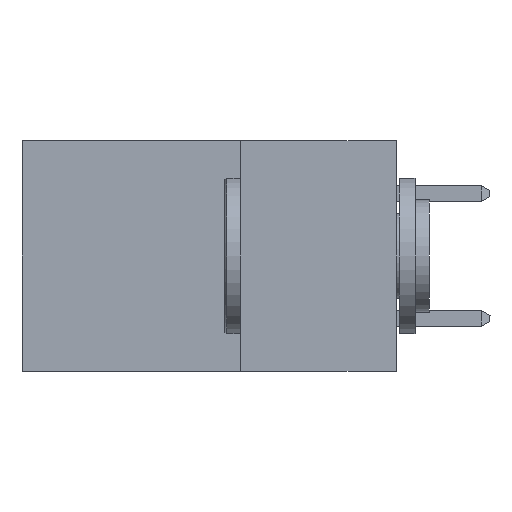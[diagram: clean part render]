
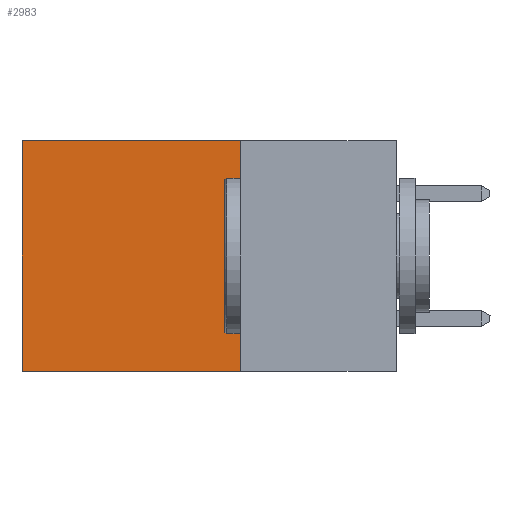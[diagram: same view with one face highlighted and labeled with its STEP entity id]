
A CAD part, left-side view. The second image highlights one B-rep face of the part: STEP entity #2983.
In plain terms, the highlighted planar face has unit normal (-1, 0, 0).
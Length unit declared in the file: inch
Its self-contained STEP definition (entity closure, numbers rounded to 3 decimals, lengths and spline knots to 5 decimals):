
#425 = EDGE_CURVE ( 'NONE', #15048, #3591, #4160, .T. ) ;
#958 = PLANE ( 'NONE',  #8337 ) ;
#1347 = EDGE_CURVE ( 'NONE', #12114, #5722, #8080, .T. ) ;
#1470 = FACE_OUTER_BOUND ( 'NONE', #16190, .T. ) ;
#1978 = CARTESIAN_POINT ( 'NONE',  ( 0.298, 0.25, 0. ) ) ;
#2418 = CARTESIAN_POINT ( 'NONE',  ( 0.298, 0.25, -0.37 ) ) ;
#2603 = VECTOR ( 'NONE', #12173, 39.37008 ) ;
#2983 = ADVANCED_FACE ( 'NONE', ( #1470 ), #958, .F. ) ;
#3263 = CARTESIAN_POINT ( 'NONE',  ( 0.298, 0.25, 0. ) ) ;
#3385 = ORIENTED_EDGE ( 'NONE', *, *, #1347, .T. ) ;
#3591 = VERTEX_POINT ( 'NONE', #10988 ) ;
#3850 = EDGE_CURVE ( 'NONE', #5722, #3591, #8456, .T. ) ;
#4106 = ORIENTED_EDGE ( 'NONE', *, *, #3850, .T. ) ;
#4160 = LINE ( 'NONE', #8777, #6154 ) ;
#4878 = ORIENTED_EDGE ( 'NONE', *, *, #15898, .F. ) ;
#5058 = DIRECTION ( 'NONE',  ( 0., 0., -1. ) ) ;
#5125 = CARTESIAN_POINT ( 'NONE',  ( 0.298, 0.25, 0. ) ) ;
#5722 = VERTEX_POINT ( 'NONE', #5901 ) ;
#5901 = CARTESIAN_POINT ( 'NONE',  ( 0.298, 0.6, 0. ) ) ;
#6154 = VECTOR ( 'NONE', #15015, 39.37008 ) ;
#7576 = LINE ( 'NONE', #3263, #2603 ) ;
#8080 = LINE ( 'NONE', #14419, #15258 ) ;
#8337 = AXIS2_PLACEMENT_3D ( 'NONE', #5125, #15247, #5058 ) ;
#8456 = LINE ( 'NONE', #14564, #9677 ) ;
#8562 = ORIENTED_EDGE ( 'NONE', *, *, #425, .F. ) ;
#8777 = CARTESIAN_POINT ( 'NONE',  ( 0.298, 0.25, -0.37 ) ) ;
#9677 = VECTOR ( 'NONE', #14897, 39.37008 ) ;
#10988 = CARTESIAN_POINT ( 'NONE',  ( 0.298, 0.6, -0.37 ) ) ;
#12114 = VERTEX_POINT ( 'NONE', #1978 ) ;
#12173 = DIRECTION ( 'NONE',  ( 0., 0., -1. ) ) ;
#14419 = CARTESIAN_POINT ( 'NONE',  ( 0.298, 0.25, 0. ) ) ;
#14564 = CARTESIAN_POINT ( 'NONE',  ( 0.298, 0.6, 0. ) ) ;
#14897 = DIRECTION ( 'NONE',  ( 0., 0., -1. ) ) ;
#15015 = DIRECTION ( 'NONE',  ( 0., 1., 0. ) ) ;
#15048 = VERTEX_POINT ( 'NONE', #2418 ) ;
#15247 = DIRECTION ( 'NONE',  ( 1., 0., 0. ) ) ;
#15258 = VECTOR ( 'NONE', #16076, 39.37008 ) ;
#15898 = EDGE_CURVE ( 'NONE', #12114, #15048, #7576, .T. ) ;
#16076 = DIRECTION ( 'NONE',  ( 0., 1., 0. ) ) ;
#16190 = EDGE_LOOP ( 'NONE', ( #4106, #8562, #4878, #3385 ) ) ;
